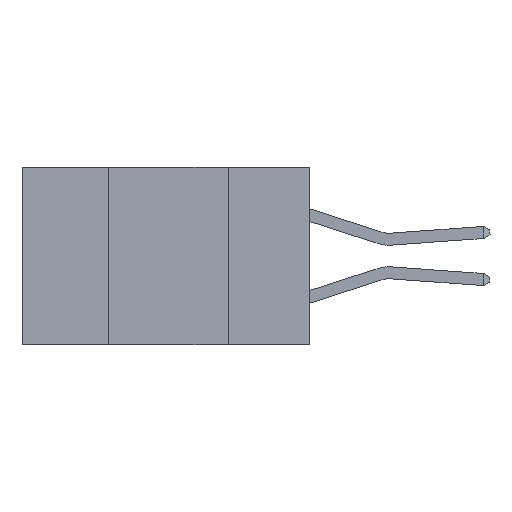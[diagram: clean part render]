
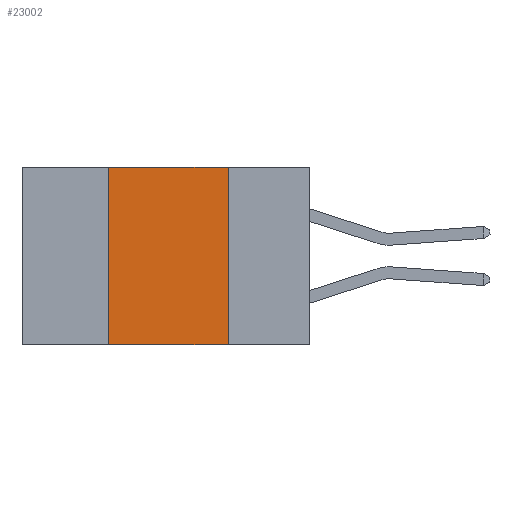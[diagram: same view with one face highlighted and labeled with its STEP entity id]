
A CAD part, left-side view. The second image highlights one B-rep face of the part: STEP entity #23002.
In plain terms, the highlighted planar face has unit normal (-1, 0, 0).
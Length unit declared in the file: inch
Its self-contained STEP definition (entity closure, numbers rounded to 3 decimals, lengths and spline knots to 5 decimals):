
#1889 = ORIENTED_EDGE ( 'NONE', *, *, #21483, .F. ) ;
#2083 = ORIENTED_EDGE ( 'NONE', *, *, #18576, .F. ) ;
#2102 = ORIENTED_EDGE ( 'NONE', *, *, #7253, .F. ) ;
#2127 = ORIENTED_EDGE ( 'NONE', *, *, #12871, .T. ) ;
#2769 = CARTESIAN_POINT ( 'NONE',  ( 0., 0.42, -0.37 ) ) ;
#3134 = FACE_OUTER_BOUND ( 'NONE', #13024, .T. ) ;
#3403 = VECTOR ( 'NONE', #13554, 39.37008 ) ;
#4751 = VECTOR ( 'NONE', #19903, 39.37008 ) ;
#7253 = EDGE_CURVE ( 'NONE', #11876, #19379, #9934, .T. ) ;
#8066 = CARTESIAN_POINT ( 'NONE',  ( 0., 0.42, 0. ) ) ;
#8608 = VERTEX_POINT ( 'NONE', #18931 ) ;
#9752 = PLANE ( 'NONE',  #21043 ) ;
#9778 = CARTESIAN_POINT ( 'NONE',  ( 0., 0.6, -0.37 ) ) ;
#9934 = LINE ( 'NONE', #8066, #19263 ) ;
#10627 = CARTESIAN_POINT ( 'NONE',  ( 0., 0.6, 0. ) ) ;
#11612 = CARTESIAN_POINT ( 'NONE',  ( 0., 0.6, 0. ) ) ;
#11702 = DIRECTION ( 'NONE',  ( 1., 0., 0. ) ) ;
#11876 = VERTEX_POINT ( 'NONE', #2769 ) ;
#12514 = DIRECTION ( 'NONE',  ( 0., -1., 0. ) ) ;
#12871 = EDGE_CURVE ( 'NONE', #11876, #8608, #18021, .T. ) ;
#13024 = EDGE_LOOP ( 'NONE', ( #1889, #2083, #2102, #2127 ) ) ;
#13124 = CARTESIAN_POINT ( 'NONE',  ( 0., 0.42, 0. ) ) ;
#13554 = DIRECTION ( 'NONE',  ( 0., -1., 0. ) ) ;
#13912 = LINE ( 'NONE', #10627, #14496 ) ;
#14496 = VECTOR ( 'NONE', #12514, 39.37008 ) ;
#14904 = DIRECTION ( 'NONE',  ( 0., 0., -1. ) ) ;
#14906 = LINE ( 'NONE', #19824, #4751 ) ;
#17550 = VERTEX_POINT ( 'NONE', #19387 ) ;
#17578 = DIRECTION ( 'NONE',  ( 0., 0., 1. ) ) ;
#18021 = LINE ( 'NONE', #9778, #3403 ) ;
#18576 = EDGE_CURVE ( 'NONE', #19379, #17550, #13912, .T. ) ;
#18931 = CARTESIAN_POINT ( 'NONE',  ( 0., 0.17, -0.37 ) ) ;
#19263 = VECTOR ( 'NONE', #17578, 39.37008 ) ;
#19379 = VERTEX_POINT ( 'NONE', #13124 ) ;
#19387 = CARTESIAN_POINT ( 'NONE',  ( 0., 0.17, 0. ) ) ;
#19824 = CARTESIAN_POINT ( 'NONE',  ( 0., 0.17, 0. ) ) ;
#19903 = DIRECTION ( 'NONE',  ( 0., 0., -1. ) ) ;
#21043 = AXIS2_PLACEMENT_3D ( 'NONE', #11612, #11702, #14904 ) ;
#21483 = EDGE_CURVE ( 'NONE', #17550, #8608, #14906, .T. ) ;
#23002 = ADVANCED_FACE ( 'NONE', ( #3134 ), #9752, .F. ) ;
